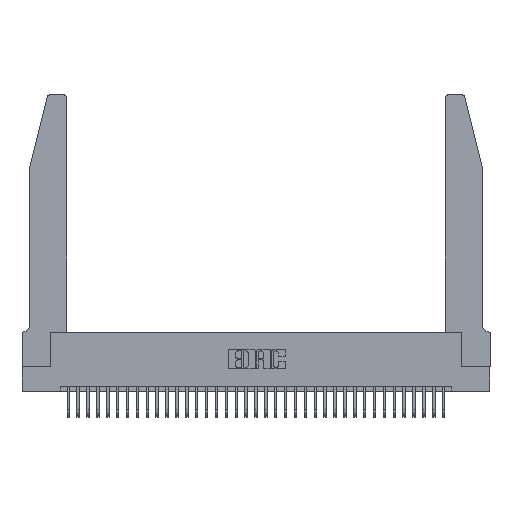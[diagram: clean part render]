
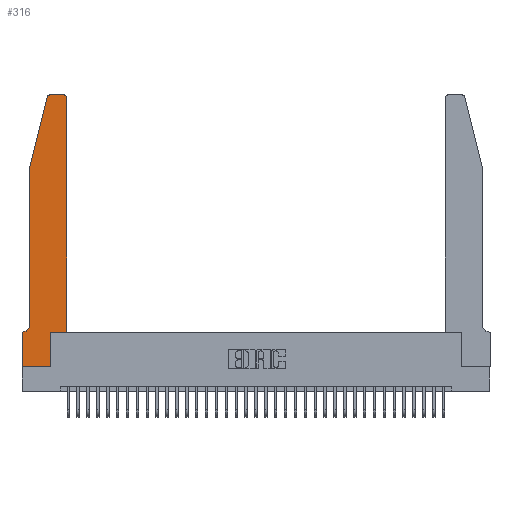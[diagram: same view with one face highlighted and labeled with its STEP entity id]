
A CAD part, top view. The second image highlights one B-rep face of the part: STEP entity #316.
In plain terms, the highlighted planar face has unit normal (0, 0, 1).
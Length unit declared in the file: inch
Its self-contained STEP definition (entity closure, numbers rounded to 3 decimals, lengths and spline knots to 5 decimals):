
#304 = AXIS2_PLACEMENT_3D ( 'NONE', #35759, #21273, #12778 ) ;
#316 = ADVANCED_FACE ( 'NONE', ( #25646 ), #4217, .T. ) ;
#494 = CARTESIAN_POINT ( 'NONE',  ( 0.4505, 0.35, 0.37 ) ) ;
#1189 = DIRECTION ( 'NONE',  ( 0., -1., 0. ) ) ;
#1869 = CARTESIAN_POINT ( 'NONE',  ( 0.0755, 2., 0.37 ) ) ;
#1949 = VERTEX_POINT ( 'NONE', #30189 ) ;
#2405 = LINE ( 'NONE', #30723, #12279 ) ;
#3116 = CARTESIAN_POINT ( 'NONE',  ( 0.0755, 0.35, 0.37 ) ) ;
#4217 = PLANE ( 'NONE',  #22865 ) ;
#4285 = CARTESIAN_POINT ( 'NONE',  ( 0., 0., 0.37 ) ) ;
#4499 = VECTOR ( 'NONE', #16801, 39.37008 ) ;
#4563 = CARTESIAN_POINT ( 'NONE',  ( 0.0055, 0.35, 0.37 ) ) ;
#5272 = LINE ( 'NONE', #494, #18362 ) ;
#6170 = ORIENTED_EDGE ( 'NONE', *, *, #13205, .T. ) ;
#6900 = DIRECTION ( 'NONE',  ( 1., 0., 0. ) ) ;
#8181 = LINE ( 'NONE', #1869, #21733 ) ;
#8349 = EDGE_CURVE ( 'NONE', #19623, #1949, #18669, .T. ) ;
#8522 = EDGE_CURVE ( 'NONE', #14596, #11156, #20523, .T. ) ;
#9349 = LINE ( 'NONE', #3116, #30198 ) ;
#10004 = AXIS2_PLACEMENT_3D ( 'NONE', #26911, #12491, #6900 ) ;
#10409 = EDGE_CURVE ( 'NONE', #1949, #21790, #32952, .T. ) ;
#10442 = ORIENTED_EDGE ( 'NONE', *, *, #34491, .T. ) ;
#10526 = CARTESIAN_POINT ( 'NONE',  ( 0.284, 2.72, 0.37 ) ) ;
#10932 = CIRCLE ( 'NONE', #10004, 0.03 ) ;
#11156 = VERTEX_POINT ( 'NONE', #27642 ) ;
#11665 = CARTESIAN_POINT ( 'NONE',  ( 0.2865, 0., 0.37 ) ) ;
#11925 = VERTEX_POINT ( 'NONE', #16259 ) ;
#12279 = VECTOR ( 'NONE', #1189, 39.37008 ) ;
#12491 = DIRECTION ( 'NONE',  ( 0., 0., 1. ) ) ;
#12621 = ORIENTED_EDGE ( 'NONE', *, *, #27787, .T. ) ;
#12778 = DIRECTION ( 'NONE',  ( -1., 0., 0. ) ) ;
#13205 = EDGE_CURVE ( 'NONE', #19938, #15183, #29182, .T. ) ;
#13258 = CARTESIAN_POINT ( 'NONE',  ( 0., 0.35, 0.37 ) ) ;
#13333 = VERTEX_POINT ( 'NONE', #19598 ) ;
#14181 = ORIENTED_EDGE ( 'NONE', *, *, #21659, .T. ) ;
#14596 = VERTEX_POINT ( 'NONE', #27096 ) ;
#14599 = EDGE_CURVE ( 'NONE', #16734, #19623, #27255, .T. ) ;
#15183 = VERTEX_POINT ( 'NONE', #4563 ) ;
#16236 = AXIS2_PLACEMENT_3D ( 'NONE', #10526, #19337, #22349 ) ;
#16259 = CARTESIAN_POINT ( 'NONE',  ( 0.4505, 2.72, 0.37 ) ) ;
#16287 = DIRECTION ( 'NONE',  ( 0., -1., 0. ) ) ;
#16495 = CARTESIAN_POINT ( 'NONE',  ( 0.2865, 0.35, 0.37 ) ) ;
#16675 = CARTESIAN_POINT ( 'NONE',  ( 0.4505, 0.35, 0.37 ) ) ;
#16734 = VERTEX_POINT ( 'NONE', #32864 ) ;
#16801 = DIRECTION ( 'NONE',  ( 1., 0., 0. ) ) ;
#17724 = DIRECTION ( 'NONE',  ( -1., 0., 0. ) ) ;
#18057 = DIRECTION ( 'NONE',  ( -1., 0., 0. ) ) ;
#18362 = VECTOR ( 'NONE', #23795, 39.37008 ) ;
#18510 = DIRECTION ( 'NONE',  ( 0., 0., 1. ) ) ;
#18669 = LINE ( 'NONE', #16495, #25979 ) ;
#18696 = CARTESIAN_POINT ( 'NONE',  ( 0.0755, 0.42, 0.37 ) ) ;
#19193 = DIRECTION ( 'NONE',  ( 1., 0., 0. ) ) ;
#19337 = DIRECTION ( 'NONE',  ( 0., 0., 1. ) ) ;
#19598 = CARTESIAN_POINT ( 'NONE',  ( 0.0755, 2., 0.37 ) ) ;
#19623 = VERTEX_POINT ( 'NONE', #11665 ) ;
#19938 = VERTEX_POINT ( 'NONE', #18696 ) ;
#20052 = DIRECTION ( 'NONE',  ( 1., 0., 0. ) ) ;
#20523 = CIRCLE ( 'NONE', #16236, 0.03 ) ;
#21273 = DIRECTION ( 'NONE',  ( 0., 0., -1. ) ) ;
#21659 = EDGE_CURVE ( 'NONE', #13333, #19938, #2405, .T. ) ;
#21726 = CARTESIAN_POINT ( 'NONE',  ( 0., 0., 0.37 ) ) ;
#21733 = VECTOR ( 'NONE', #22123, 39.37008 ) ;
#21790 = VERTEX_POINT ( 'NONE', #25977 ) ;
#22123 = DIRECTION ( 'NONE',  ( -0.239, -0.971, 0. ) ) ;
#22349 = DIRECTION ( 'NONE',  ( 1., 0., 0. ) ) ;
#22831 = EDGE_CURVE ( 'NONE', #23467, #16734, #29389, .T. ) ;
#22844 = EDGE_CURVE ( 'NONE', #11156, #13333, #8181, .T. ) ;
#22865 = AXIS2_PLACEMENT_3D ( 'NONE', #35797, #18510, #19193 ) ;
#22955 = VECTOR ( 'NONE', #18057, 39.37008 ) ;
#23404 = LINE ( 'NONE', #24133, #22955 ) ;
#23467 = VERTEX_POINT ( 'NONE', #13258 ) ;
#23795 = DIRECTION ( 'NONE',  ( 0., 1., 0. ) ) ;
#24133 = CARTESIAN_POINT ( 'NONE',  ( 0.2605, 2.75, 0.37 ) ) ;
#24395 = ORIENTED_EDGE ( 'NONE', *, *, #28593, .T. ) ;
#25416 = CARTESIAN_POINT ( 'NONE',  ( 0.4205, 2.75, 0.37 ) ) ;
#25646 = FACE_OUTER_BOUND ( 'NONE', #29902, .T. ) ;
#25977 = CARTESIAN_POINT ( 'NONE',  ( 0.4505, 0.35, 0.37 ) ) ;
#25979 = VECTOR ( 'NONE', #34909, 39.37008 ) ;
#26028 = ORIENTED_EDGE ( 'NONE', *, *, #14599, .T. ) ;
#26911 = CARTESIAN_POINT ( 'NONE',  ( 0.4205, 2.72, 0.37 ) ) ;
#27096 = CARTESIAN_POINT ( 'NONE',  ( 0.284, 2.75, 0.37 ) ) ;
#27255 = LINE ( 'NONE', #4285, #34071 ) ;
#27642 = CARTESIAN_POINT ( 'NONE',  ( 0.25487, 2.72718, 0.37 ) ) ;
#27787 = EDGE_CURVE ( 'NONE', #21790, #11925, #5272, .T. ) ;
#27957 = ORIENTED_EDGE ( 'NONE', *, *, #8349, .T. ) ;
#28593 = EDGE_CURVE ( 'NONE', #36994, #14596, #23404, .T. ) ;
#29034 = ORIENTED_EDGE ( 'NONE', *, *, #22844, .T. ) ;
#29182 = CIRCLE ( 'NONE', #304, 0.07 ) ;
#29255 = ORIENTED_EDGE ( 'NONE', *, *, #8522, .T. ) ;
#29389 = LINE ( 'NONE', #21726, #34417 ) ;
#29902 = EDGE_LOOP ( 'NONE', ( #24395, #29255, #29034, #14181, #6170, #10442, #32241, #26028, #27957, #36932, #12621, #31668 ) ) ;
#30189 = CARTESIAN_POINT ( 'NONE',  ( 0.2865, 0.35, 0.37 ) ) ;
#30198 = VECTOR ( 'NONE', #17724, 39.37008 ) ;
#30723 = CARTESIAN_POINT ( 'NONE',  ( 0.0755, 2., 0.37 ) ) ;
#31668 = ORIENTED_EDGE ( 'NONE', *, *, #35338, .T. ) ;
#32241 = ORIENTED_EDGE ( 'NONE', *, *, #22831, .T. ) ;
#32864 = CARTESIAN_POINT ( 'NONE',  ( 0., 0., 0.37 ) ) ;
#32952 = LINE ( 'NONE', #16675, #4499 ) ;
#34071 = VECTOR ( 'NONE', #20052, 39.37008 ) ;
#34417 = VECTOR ( 'NONE', #16287, 39.37008 ) ;
#34491 = EDGE_CURVE ( 'NONE', #15183, #23467, #9349, .T. ) ;
#34909 = DIRECTION ( 'NONE',  ( 0., 1., 0. ) ) ;
#35338 = EDGE_CURVE ( 'NONE', #11925, #36994, #10932, .T. ) ;
#35759 = CARTESIAN_POINT ( 'NONE',  ( 0.0055, 0.42, 0.37 ) ) ;
#35797 = CARTESIAN_POINT ( 'NONE',  ( 0., 0.35, 0.37 ) ) ;
#36932 = ORIENTED_EDGE ( 'NONE', *, *, #10409, .T. ) ;
#36994 = VERTEX_POINT ( 'NONE', #25416 ) ;
